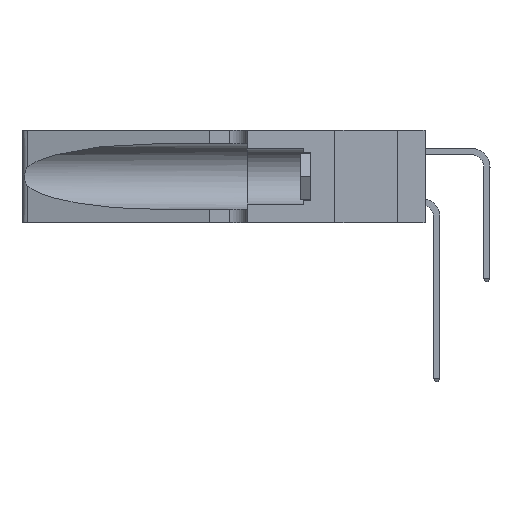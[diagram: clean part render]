
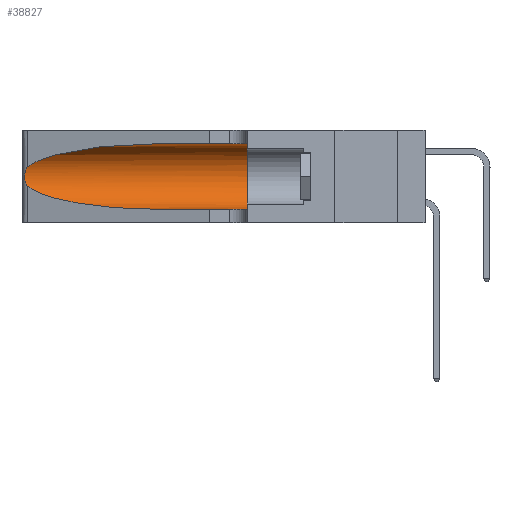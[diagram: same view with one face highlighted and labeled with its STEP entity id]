
A CAD part, left-side view. The second image highlights one B-rep face of the part: STEP entity #38827.
In plain terms, the highlighted cylindrical face has radius 3.308 mm (diameter 6.617 mm), a partial arc.
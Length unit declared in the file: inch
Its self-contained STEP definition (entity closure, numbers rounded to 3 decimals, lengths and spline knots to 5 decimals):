
#431 = CARTESIAN_POINT ( 'NONE',  ( 0.25555, 1.22994, 0.2215 ) ) ;
#582 = CARTESIAN_POINT ( 'NONE',  ( 0.25854, 1.2359, 0.20912 ) ) ;
#1917 = EDGE_CURVE ( 'NONE', #9509, #5093, #8737, .T. ) ;
#3598 = CARTESIAN_POINT ( 'NONE',  ( 0.2373, 1.15595, 0.08982 ) ) ;
#3869 = DIRECTION ( 'NONE',  ( 0., 1., 0. ) ) ;
#4144 = CARTESIAN_POINT ( 'NONE',  ( 0.26075, 1.23896, 0.19203 ) ) ;
#4375 = FACE_OUTER_BOUND ( 'NONE', #12302, .T. ) ;
#5093 = VERTEX_POINT ( 'NONE', #14418 ) ;
#6536 = DIRECTION ( 'NONE',  ( 0., 0., -1. ) ) ;
#7658 = CARTESIAN_POINT ( 'NONE',  ( 0.26017, 1.23833, 0.17102 ) ) ;
#8017 = LINE ( 'NONE', #26307, #34937 ) ;
#8588 = CARTESIAN_POINT ( 'NONE',  ( 0.2373, 1.15595, 0.28018 ) ) ;
#8737 =( BOUNDED_CURVE ( )  B_SPLINE_CURVE ( 3, ( #31671, #3598, #24656, #10617 ),
 .UNSPECIFIED., .F., .F. ) 
 B_SPLINE_CURVE_WITH_KNOTS ( ( 4, 4 ),
 ( 3.44316, 4.71239 ),
 .UNSPECIFIED. ) 
 CURVE ( )  GEOMETRIC_REPRESENTATION_ITEM ( )  RATIONAL_B_SPLINE_CURVE ( ( 1., 0.87, 0.87, 1. ) ) 
 REPRESENTATION_ITEM ( '' )  );
#9509 = VERTEX_POINT ( 'NONE', #14812 ) ;
#9978 = ORIENTED_EDGE ( 'NONE', *, *, #24462, .F. ) ;
#9988 = EDGE_CURVE ( 'NONE', #27484, #23110, #23195, .T. ) ;
#10617 = CARTESIAN_POINT ( 'NONE',  ( 0.1305, 0.72297, 0.05475 ) ) ;
#11193 = CARTESIAN_POINT ( 'NONE',  ( 0.25789, 1.23486, 0.15765 ) ) ;
#11558 = CARTESIAN_POINT ( 'NONE',  ( 0.25487, 1.22718, 0.22369 ) ) ;
#12302 = EDGE_LOOP ( 'NONE', ( #30329, #41750, #33634, #16109, #36917, #9978 ) ) ;
#14418 = CARTESIAN_POINT ( 'NONE',  ( 0.1305, 0.72297, 0.05475 ) ) ;
#14674 = CARTESIAN_POINT ( 'NONE',  ( 0.1305, 0.35, 0.31525 ) ) ;
#14757 = CARTESIAN_POINT ( 'NONE',  ( 0.25555, 1.22993, 0.14849 ) ) ;
#14812 = CARTESIAN_POINT ( 'NONE',  ( 0.25487, 1.22718, 0.14631 ) ) ;
#16109 = ORIENTED_EDGE ( 'NONE', *, *, #26791, .T. ) ;
#17337 =( BOUNDED_CURVE ( )  B_SPLINE_CURVE ( 3, ( #26289, #40141, #8588, #29789 ),
 .UNSPECIFIED., .F., .F. ) 
 B_SPLINE_CURVE_WITH_KNOTS ( ( 4, 4 ),
 ( 1.5708, 2.84003 ),
 .UNSPECIFIED. ) 
 CURVE ( )  GEOMETRIC_REPRESENTATION_ITEM ( )  RATIONAL_B_SPLINE_CURVE ( ( 1., 0.87, 0.87, 1. ) ) 
 REPRESENTATION_ITEM ( '' )  );
#18011 = CARTESIAN_POINT ( 'NONE',  ( 0.25487, 1.22718, 0.22369 ) ) ;
#20570 = DIRECTION ( 'NONE',  ( 0., -1., 0. ) ) ;
#21035 = VECTOR ( 'NONE', #42680, 39.37008 ) ;
#21695 = CARTESIAN_POINT ( 'NONE',  ( 0.25787, 1.23484, 0.2124 ) ) ;
#23110 = VERTEX_POINT ( 'NONE', #43763 ) ;
#23195 = CIRCLE ( 'NONE', #39360, 0.13025 ) ;
#24462 = EDGE_CURVE ( 'NONE', #29232, #27484, #8017, .T. ) ;
#24656 = CARTESIAN_POINT ( 'NONE',  ( 0.18966, 0.96281, 0.05475 ) ) ;
#24942 = CARTESIAN_POINT ( 'NONE',  ( 0.1305, 0.35, 0.185 ) ) ;
#25222 = CARTESIAN_POINT ( 'NONE',  ( 0.26018, 1.23835, 0.19895 ) ) ;
#26154 = CARTESIAN_POINT ( 'NONE',  ( 0.1305, 0.72297, 0.31525 ) ) ;
#26289 = CARTESIAN_POINT ( 'NONE',  ( 0.1305, 0.72297, 0.31525 ) ) ;
#26307 = CARTESIAN_POINT ( 'NONE',  ( 0.1305, 1.61858, 0.31525 ) ) ;
#26346 = EDGE_CURVE ( 'NONE', #29232, #42169, #17337, .T. ) ;
#26791 = EDGE_CURVE ( 'NONE', #5093, #23110, #39592, .T. ) ;
#27484 = VERTEX_POINT ( 'NONE', #14674 ) ;
#27584 = CARTESIAN_POINT ( 'NONE',  ( 0.1305, 1.61858, 0.185 ) ) ;
#28428 = DIRECTION ( 'NONE',  ( 0., 0., 1. ) ) ;
#28715 = CARTESIAN_POINT ( 'NONE',  ( 0.26075, 1.23896, 0.178 ) ) ;
#29232 = VERTEX_POINT ( 'NONE', #26154 ) ;
#29789 = CARTESIAN_POINT ( 'NONE',  ( 0.25487, 1.22718, 0.22369 ) ) ;
#30110 = AXIS2_PLACEMENT_3D ( 'NONE', #27584, #20570, #6536 ) ;
#30329 = ORIENTED_EDGE ( 'NONE', *, *, #26346, .T. ) ;
#31285 = CYLINDRICAL_SURFACE ( 'NONE', #30110, 0.13025 ) ;
#31671 = CARTESIAN_POINT ( 'NONE',  ( 0.25487, 1.22718, 0.14631 ) ) ;
#32233 = CARTESIAN_POINT ( 'NONE',  ( 0.25856, 1.23593, 0.16098 ) ) ;
#33340 = DIRECTION ( 'NONE',  ( 0., -1., 0. ) ) ;
#33634 = ORIENTED_EDGE ( 'NONE', *, *, #1917, .T. ) ;
#34937 = VECTOR ( 'NONE', #33340, 39.37008 ) ;
#35756 = CARTESIAN_POINT ( 'NONE',  ( 0.25639, 1.23186, 0.15144 ) ) ;
#36917 = ORIENTED_EDGE ( 'NONE', *, *, #9988, .F. ) ;
#38827 = ADVANCED_FACE ( 'NONE', ( #4375 ), #31285, .F. ) ;
#39202 = CARTESIAN_POINT ( 'NONE',  ( 0.1305, 1.61858, 0.05475 ) ) ;
#39230 = CARTESIAN_POINT ( 'NONE',  ( 0.25487, 1.22718, 0.14631 ) ) ;
#39360 = AXIS2_PLACEMENT_3D ( 'NONE', #24942, #3869, #28428 ) ;
#39592 = LINE ( 'NONE', #39202, #21035 ) ;
#40141 = CARTESIAN_POINT ( 'NONE',  ( 0.18966, 0.96281, 0.31525 ) ) ;
#40809 = EDGE_CURVE ( 'NONE', #42169, #9509, #41557, .T. ) ;
#41557 = B_SPLINE_CURVE_WITH_KNOTS ( 'NONE', 3,
 ( #18011, #431, #42555, #21695, #582, #25222, #4144, #28715, #7658, #32233, #11193, #35756, #14757, #39230 ),
 .UNSPECIFIED., .F., .F.,
 ( 4, 2, 2, 2, 2, 2, 4 ),
 ( 0., 0.00027, 0.00053, 0.00107, 0.0016, 0.00187, 0.00214 ),
 .UNSPECIFIED. ) ;
#41750 = ORIENTED_EDGE ( 'NONE', *, *, #40809, .T. ) ;
#42169 = VERTEX_POINT ( 'NONE', #11558 ) ;
#42555 = CARTESIAN_POINT ( 'NONE',  ( 0.25639, 1.23184, 0.21858 ) ) ;
#42680 = DIRECTION ( 'NONE',  ( 0., -1., 0. ) ) ;
#43763 = CARTESIAN_POINT ( 'NONE',  ( 0.1305, 0.35, 0.05475 ) ) ;
